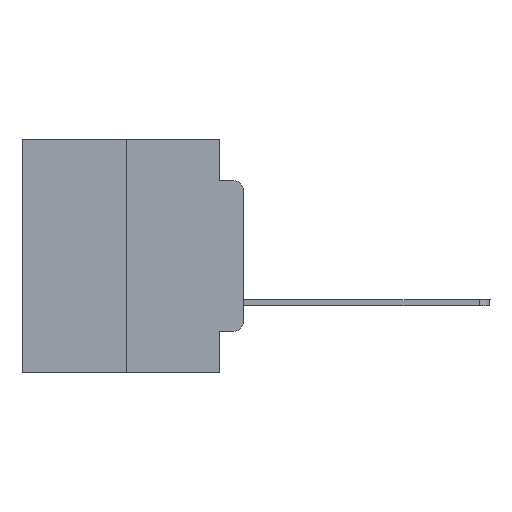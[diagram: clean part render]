
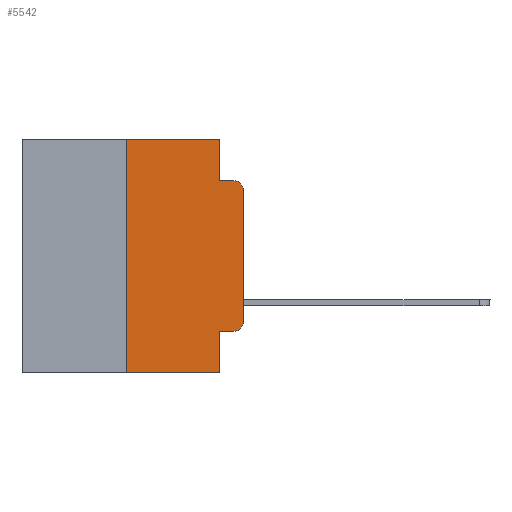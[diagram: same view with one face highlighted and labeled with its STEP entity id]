
A CAD part, left-side view. The second image highlights one B-rep face of the part: STEP entity #5542.
In plain terms, the highlighted planar face has unit normal (-1, 0, 0).
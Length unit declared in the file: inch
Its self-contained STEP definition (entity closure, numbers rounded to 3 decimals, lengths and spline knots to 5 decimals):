
#527 = CARTESIAN_POINT ( 'NONE',  ( 0., 0.051, -0.0885 ) ) ;
#1199 = VERTEX_POINT ( 'NONE', #6538 ) ;
#1204 = CARTESIAN_POINT ( 'NONE',  ( 0., 0.051, -0.5 ) ) ;
#2012 = ORIENTED_EDGE ( 'NONE', *, *, #22720, .T. ) ;
#2161 = DIRECTION ( 'NONE',  ( 0., 0., -1. ) ) ;
#2311 = DIRECTION ( 'NONE',  ( -1., 0., 0. ) ) ;
#2849 = FACE_OUTER_BOUND ( 'NONE', #11824, .T. ) ;
#3204 = LINE ( 'NONE', #17427, #26914 ) ;
#3839 = VERTEX_POINT ( 'NONE', #1204 ) ;
#3895 = DIRECTION ( 'NONE',  ( 0., 0., 1. ) ) ;
#4034 = DIRECTION ( 'NONE',  ( 0., 0., -1. ) ) ;
#4724 = EDGE_CURVE ( 'NONE', #16050, #19997, #6195, .T. ) ;
#4770 = ORIENTED_EDGE ( 'NONE', *, *, #23895, .F. ) ;
#4879 = LINE ( 'NONE', #26403, #21586 ) ;
#5017 = ORIENTED_EDGE ( 'NONE', *, *, #15953, .T. ) ;
#5306 = CARTESIAN_POINT ( 'NONE',  ( 0., 0., -0.1085 ) ) ;
#5542 = ADVANCED_FACE ( 'NONE', ( #2849 ), #16929, .F. ) ;
#5618 = DIRECTION ( 'NONE',  ( 0., -1., 0. ) ) ;
#5740 = VECTOR ( 'NONE', #12419, 39.37008 ) ;
#5758 = VECTOR ( 'NONE', #4034, 39.37008 ) ;
#5910 = VERTEX_POINT ( 'NONE', #25969 ) ;
#6195 = LINE ( 'NONE', #6495, #26224 ) ;
#6320 = ORIENTED_EDGE ( 'NONE', *, *, #12134, .F. ) ;
#6322 = DIRECTION ( 'NONE',  ( 0., -1., 0. ) ) ;
#6332 = VECTOR ( 'NONE', #2161, 39.37008 ) ;
#6349 = CARTESIAN_POINT ( 'NONE',  ( 0., 0.051, 0. ) ) ;
#6495 = CARTESIAN_POINT ( 'NONE',  ( 0., 0.051, -0.0885 ) ) ;
#6538 = CARTESIAN_POINT ( 'NONE',  ( 0., 0.02, -0.4115 ) ) ;
#6727 = EDGE_CURVE ( 'NONE', #14918, #12495, #21136, .T. ) ;
#8916 = VECTOR ( 'NONE', #5618, 39.37008 ) ;
#9086 = ORIENTED_EDGE ( 'NONE', *, *, #18984, .T. ) ;
#9143 = EDGE_CURVE ( 'NONE', #19130, #3839, #24991, .T. ) ;
#9773 = CIRCLE ( 'NONE', #23515, 0.02 ) ;
#10711 = ORIENTED_EDGE ( 'NONE', *, *, #6727, .T. ) ;
#11278 = CARTESIAN_POINT ( 'NONE',  ( 0., 0.25, -0.5 ) ) ;
#11824 = EDGE_LOOP ( 'NONE', ( #10711, #5017, #24656, #17740, #4770, #13830, #24188, #6320, #2012, #9086 ) ) ;
#12018 = LINE ( 'NONE', #12722, #6332 ) ;
#12134 = EDGE_CURVE ( 'NONE', #5910, #3839, #17128, .T. ) ;
#12175 = DIRECTION ( 'NONE',  ( 1., 0., 0. ) ) ;
#12281 = CARTESIAN_POINT ( 'NONE',  ( 0., 0.25, 0. ) ) ;
#12419 = DIRECTION ( 'NONE',  ( 0., 0., 1. ) ) ;
#12495 = VERTEX_POINT ( 'NONE', #5306 ) ;
#12532 = DIRECTION ( 'NONE',  ( 0., 0., -1. ) ) ;
#12722 = CARTESIAN_POINT ( 'NONE',  ( 0., 0.051, 0. ) ) ;
#13733 = AXIS2_PLACEMENT_3D ( 'NONE', #23101, #12175, #14289 ) ;
#13830 = ORIENTED_EDGE ( 'NONE', *, *, #23014, .F. ) ;
#14289 = DIRECTION ( 'NONE',  ( 0., 0., -1. ) ) ;
#14589 = EDGE_CURVE ( 'NONE', #27197, #16050, #12018, .T. ) ;
#14918 = VERTEX_POINT ( 'NONE', #21917 ) ;
#15110 = DIRECTION ( 'NONE',  ( 0., 0., -1. ) ) ;
#15306 = VERTEX_POINT ( 'NONE', #17498 ) ;
#15927 = AXIS2_PLACEMENT_3D ( 'NONE', #23381, #2311, #12532 ) ;
#15953 = EDGE_CURVE ( 'NONE', #12495, #19997, #21932, .T. ) ;
#16050 = VERTEX_POINT ( 'NONE', #527 ) ;
#16929 = PLANE ( 'NONE',  #13733 ) ;
#17128 = LINE ( 'NONE', #6349, #5758 ) ;
#17427 = CARTESIAN_POINT ( 'NONE',  ( 0., 0.473, 0. ) ) ;
#17498 = CARTESIAN_POINT ( 'NONE',  ( 0., 0.25, 0. ) ) ;
#17740 = ORIENTED_EDGE ( 'NONE', *, *, #14589, .F. ) ;
#18442 = CARTESIAN_POINT ( 'NONE',  ( 0., 0.02, -0.0885 ) ) ;
#18984 = EDGE_CURVE ( 'NONE', #1199, #14918, #9773, .T. ) ;
#19130 = VERTEX_POINT ( 'NONE', #11278 ) ;
#19262 = DIRECTION ( 'NONE',  ( -1., 0., 0. ) ) ;
#19997 = VERTEX_POINT ( 'NONE', #18442 ) ;
#20128 = DIRECTION ( 'NONE',  ( 0., -1., 0. ) ) ;
#20551 = CARTESIAN_POINT ( 'NONE',  ( 0., 0., 0. ) ) ;
#20940 = VECTOR ( 'NONE', #3895, 39.37008 ) ;
#21136 = LINE ( 'NONE', #20551, #5740 ) ;
#21586 = VECTOR ( 'NONE', #20128, 39.37008 ) ;
#21917 = CARTESIAN_POINT ( 'NONE',  ( 0., 0., -0.3915 ) ) ;
#21932 = CIRCLE ( 'NONE', #15927, 0.02 ) ;
#22720 = EDGE_CURVE ( 'NONE', #5910, #1199, #4879, .T. ) ;
#22920 = CARTESIAN_POINT ( 'NONE',  ( 0., 0.473, -0.5 ) ) ;
#23014 = EDGE_CURVE ( 'NONE', #19130, #15306, #23935, .T. ) ;
#23101 = CARTESIAN_POINT ( 'NONE',  ( 0., 0.473, 0. ) ) ;
#23381 = CARTESIAN_POINT ( 'NONE',  ( 0., 0.02, -0.1085 ) ) ;
#23515 = AXIS2_PLACEMENT_3D ( 'NONE', #23540, #19262, #15110 ) ;
#23540 = CARTESIAN_POINT ( 'NONE',  ( 0., 0.02, -0.3915 ) ) ;
#23785 = DIRECTION ( 'NONE',  ( 0., -1., 0. ) ) ;
#23895 = EDGE_CURVE ( 'NONE', #15306, #27197, #3204, .T. ) ;
#23935 = LINE ( 'NONE', #12281, #20940 ) ;
#24188 = ORIENTED_EDGE ( 'NONE', *, *, #9143, .T. ) ;
#24290 = CARTESIAN_POINT ( 'NONE',  ( 0., 0.051, 0. ) ) ;
#24656 = ORIENTED_EDGE ( 'NONE', *, *, #4724, .F. ) ;
#24991 = LINE ( 'NONE', #22920, #8916 ) ;
#25969 = CARTESIAN_POINT ( 'NONE',  ( 0., 0.051, -0.4115 ) ) ;
#26224 = VECTOR ( 'NONE', #6322, 39.37008 ) ;
#26403 = CARTESIAN_POINT ( 'NONE',  ( 0., 0.051, -0.4115 ) ) ;
#26914 = VECTOR ( 'NONE', #23785, 39.37008 ) ;
#27197 = VERTEX_POINT ( 'NONE', #24290 ) ;
